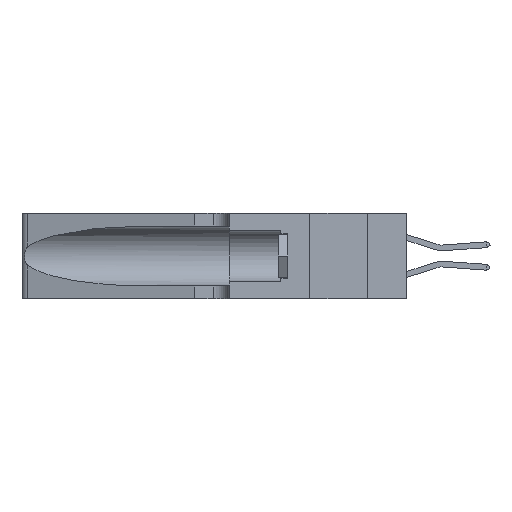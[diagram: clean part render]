
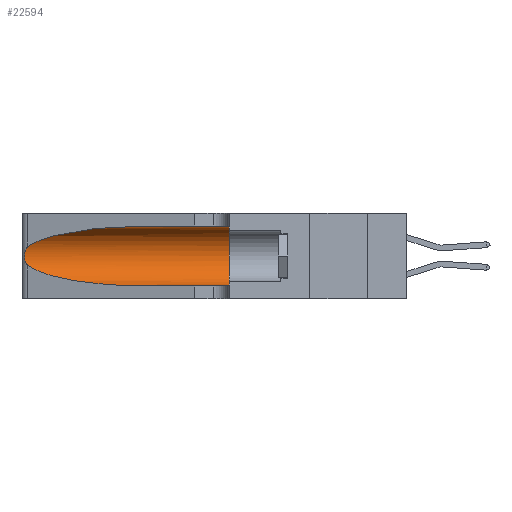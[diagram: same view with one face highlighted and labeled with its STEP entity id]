
A CAD part, left-side view. The second image highlights one B-rep face of the part: STEP entity #22594.
In plain terms, the highlighted cylindrical face has radius 3.308 mm (diameter 6.617 mm), a partial arc.
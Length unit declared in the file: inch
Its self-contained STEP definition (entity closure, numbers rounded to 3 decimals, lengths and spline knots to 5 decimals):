
#594 = CARTESIAN_POINT ( 'NONE',  ( 0.1305, 0.72297, 0.31525 ) ) ;
#2640 = CARTESIAN_POINT ( 'NONE',  ( 0.2373, 1.15595, 0.08982 ) ) ;
#2687 = VECTOR ( 'NONE', #20321, 39.37008 ) ;
#3247 = DIRECTION ( 'NONE',  ( 0., -1., 0. ) ) ;
#3853 = CARTESIAN_POINT ( 'NONE',  ( 0.1305, 0.72297, 0.31525 ) ) ;
#3858 = CARTESIAN_POINT ( 'NONE',  ( 0.25854, 1.2359, 0.20912 ) ) ;
#4282 = CARTESIAN_POINT ( 'NONE',  ( 0.25487, 1.22718, 0.22369 ) ) ;
#4315 = CARTESIAN_POINT ( 'NONE',  ( 0.1305, 0.35, 0.31525 ) ) ;
#4981 = AXIS2_PLACEMENT_3D ( 'NONE', #20399, #31956, #14388 ) ;
#5880 = EDGE_CURVE ( 'NONE', #10499, #37789, #26044, .T. ) ;
#6478 = CARTESIAN_POINT ( 'NONE',  ( 0.25487, 1.22718, 0.22369 ) ) ;
#7885 = VECTOR ( 'NONE', #3247, 39.37008 ) ;
#7955 = CARTESIAN_POINT ( 'NONE',  ( 0.18966, 0.96281, 0.05475 ) ) ;
#9302 = CARTESIAN_POINT ( 'NONE',  ( 0.26075, 1.23896, 0.178 ) ) ;
#9972 = EDGE_CURVE ( 'NONE', #14768, #10499, #35982, .T. ) ;
#10327 = EDGE_LOOP ( 'NONE', ( #31414, #18901, #26108, #16967, #16066, #22181 ) ) ;
#10499 = VERTEX_POINT ( 'NONE', #18817 ) ;
#12154 = EDGE_CURVE ( 'NONE', #16473, #30981, #22324, .T. ) ;
#12363 = CARTESIAN_POINT ( 'NONE',  ( 0.25639, 1.23186, 0.15144 ) ) ;
#13290 = CIRCLE ( 'NONE', #4981, 0.13025 ) ;
#14388 = DIRECTION ( 'NONE',  ( 0., 0., 1. ) ) ;
#14434 = CARTESIAN_POINT ( 'NONE',  ( 0.1305, 1.61858, 0.05475 ) ) ;
#14768 = VERTEX_POINT ( 'NONE', #31616 ) ;
#14945 = CARTESIAN_POINT ( 'NONE',  ( 0.25789, 1.23486, 0.15765 ) ) ;
#14981 = CARTESIAN_POINT ( 'NONE',  ( 0.26018, 1.23835, 0.19895 ) ) ;
#16066 = ORIENTED_EDGE ( 'NONE', *, *, #18561, .F. ) ;
#16473 = VERTEX_POINT ( 'NONE', #3853 ) ;
#16967 = ORIENTED_EDGE ( 'NONE', *, *, #5880, .T. ) ;
#17073 = CARTESIAN_POINT ( 'NONE',  ( 0.1305, 0.72297, 0.05475 ) ) ;
#17553 = LINE ( 'NONE', #26662, #7885 ) ;
#18272 = CARTESIAN_POINT ( 'NONE',  ( 0.25487, 1.22718, 0.14631 ) ) ;
#18561 = EDGE_CURVE ( 'NONE', #32714, #37789, #13290, .T. ) ;
#18817 = CARTESIAN_POINT ( 'NONE',  ( 0.1305, 0.72297, 0.05475 ) ) ;
#18901 = ORIENTED_EDGE ( 'NONE', *, *, #19550, .T. ) ;
#19286 = DIRECTION ( 'NONE',  ( 0., 0., -1. ) ) ;
#19550 = EDGE_CURVE ( 'NONE', #30981, #14768, #26335, .T. ) ;
#20321 = DIRECTION ( 'NONE',  ( 0., -1., 0. ) ) ;
#20399 = CARTESIAN_POINT ( 'NONE',  ( 0.1305, 0.35, 0.185 ) ) ;
#20619 = CARTESIAN_POINT ( 'NONE',  ( 0.2373, 1.15595, 0.28018 ) ) ;
#21118 = CARTESIAN_POINT ( 'NONE',  ( 0.18966, 0.96281, 0.31525 ) ) ;
#21254 = AXIS2_PLACEMENT_3D ( 'NONE', #27861, #33950, #19286 ) ;
#22181 = ORIENTED_EDGE ( 'NONE', *, *, #33834, .F. ) ;
#22324 =( BOUNDED_CURVE ( )  B_SPLINE_CURVE ( 3, ( #594, #21118, #20619, #6478 ),
 .UNSPECIFIED., .F., .F. ) 
 B_SPLINE_CURVE_WITH_KNOTS ( ( 4, 4 ),
 ( 1.5708, 2.84003 ),
 .UNSPECIFIED. ) 
 CURVE ( )  GEOMETRIC_REPRESENTATION_ITEM ( )  RATIONAL_B_SPLINE_CURVE ( ( 1., 0.87, 0.87, 1. ) ) 
 REPRESENTATION_ITEM ( '' )  );
#22594 = ADVANCED_FACE ( 'NONE', ( #30410 ), #26715, .F. ) ;
#22974 = CARTESIAN_POINT ( 'NONE',  ( 0.25487, 1.22718, 0.14631 ) ) ;
#24771 = CARTESIAN_POINT ( 'NONE',  ( 0.25555, 1.22994, 0.2215 ) ) ;
#25869 = CARTESIAN_POINT ( 'NONE',  ( 0.25639, 1.23184, 0.21858 ) ) ;
#26044 = LINE ( 'NONE', #14434, #2687 ) ;
#26108 = ORIENTED_EDGE ( 'NONE', *, *, #9972, .T. ) ;
#26335 = B_SPLINE_CURVE_WITH_KNOTS ( 'NONE', 3,
 ( #4282, #24771, #25869, #34413, #3858, #14981, #29570, #9302, #30085, #26736, #14945, #12363, #32903, #18272 ),
 .UNSPECIFIED., .F., .F.,
 ( 4, 2, 2, 2, 2, 2, 4 ),
 ( 0., 0.00027, 0.00053, 0.00107, 0.0016, 0.00187, 0.00214 ),
 .UNSPECIFIED. ) ;
#26662 = CARTESIAN_POINT ( 'NONE',  ( 0.1305, 1.61858, 0.31525 ) ) ;
#26715 = CYLINDRICAL_SURFACE ( 'NONE', #21254, 0.13025 ) ;
#26736 = CARTESIAN_POINT ( 'NONE',  ( 0.25856, 1.23593, 0.16098 ) ) ;
#27861 = CARTESIAN_POINT ( 'NONE',  ( 0.1305, 1.61858, 0.185 ) ) ;
#29570 = CARTESIAN_POINT ( 'NONE',  ( 0.26075, 1.23896, 0.19203 ) ) ;
#30085 = CARTESIAN_POINT ( 'NONE',  ( 0.26017, 1.23833, 0.17102 ) ) ;
#30410 = FACE_OUTER_BOUND ( 'NONE', #10327, .T. ) ;
#30981 = VERTEX_POINT ( 'NONE', #35907 ) ;
#31414 = ORIENTED_EDGE ( 'NONE', *, *, #12154, .T. ) ;
#31616 = CARTESIAN_POINT ( 'NONE',  ( 0.25487, 1.22718, 0.14631 ) ) ;
#31956 = DIRECTION ( 'NONE',  ( 0., 1., 0. ) ) ;
#32714 = VERTEX_POINT ( 'NONE', #4315 ) ;
#32903 = CARTESIAN_POINT ( 'NONE',  ( 0.25555, 1.22993, 0.14849 ) ) ;
#33834 = EDGE_CURVE ( 'NONE', #16473, #32714, #17553, .T. ) ;
#33950 = DIRECTION ( 'NONE',  ( 0., -1., 0. ) ) ;
#34413 = CARTESIAN_POINT ( 'NONE',  ( 0.25787, 1.23484, 0.2124 ) ) ;
#35906 = CARTESIAN_POINT ( 'NONE',  ( 0.1305, 0.35, 0.05475 ) ) ;
#35907 = CARTESIAN_POINT ( 'NONE',  ( 0.25487, 1.22718, 0.22369 ) ) ;
#35982 =( BOUNDED_CURVE ( )  B_SPLINE_CURVE ( 3, ( #22974, #2640, #7955, #17073 ),
 .UNSPECIFIED., .F., .T. ) 
 B_SPLINE_CURVE_WITH_KNOTS ( ( 4, 4 ),
 ( 3.44316, 4.71239 ),
 .UNSPECIFIED. ) 
 CURVE ( )  GEOMETRIC_REPRESENTATION_ITEM ( )  RATIONAL_B_SPLINE_CURVE ( ( 1., 0.87, 0.87, 1. ) ) 
 REPRESENTATION_ITEM ( '' )  );
#37789 = VERTEX_POINT ( 'NONE', #35906 ) ;
